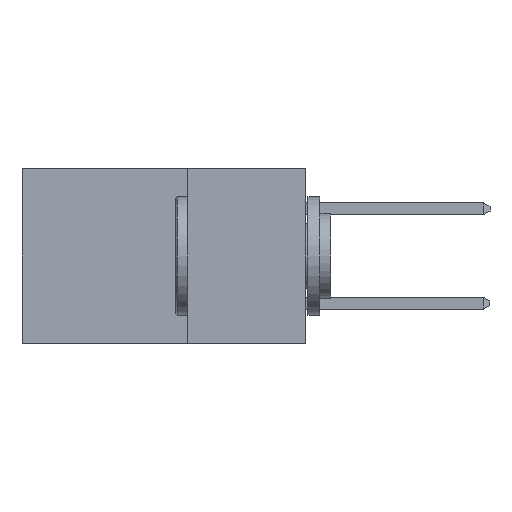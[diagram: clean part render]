
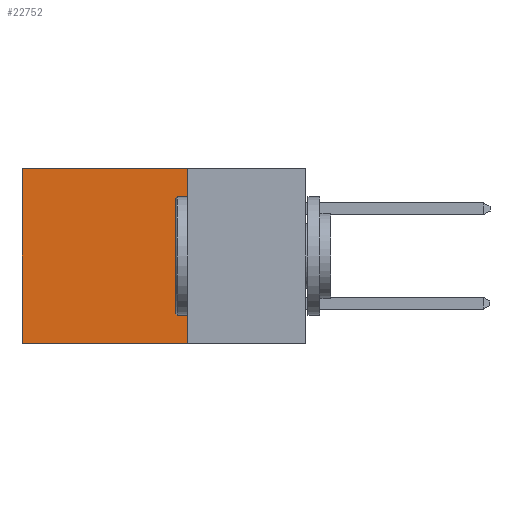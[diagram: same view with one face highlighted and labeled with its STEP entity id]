
A CAD part, left-side view. The second image highlights one B-rep face of the part: STEP entity #22752.
In plain terms, the highlighted planar face has unit normal (-1, 0, 0).
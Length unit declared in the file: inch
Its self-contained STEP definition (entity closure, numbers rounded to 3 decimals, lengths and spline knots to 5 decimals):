
#665 = LINE ( 'NONE', #20481, #9593 ) ;
#2445 = VERTEX_POINT ( 'NONE', #21911 ) ;
#3149 = LINE ( 'NONE', #11725, #16633 ) ;
#3581 = VERTEX_POINT ( 'NONE', #5821 ) ;
#3731 = EDGE_LOOP ( 'NONE', ( #21930, #4913, #4313, #12067 ) ) ;
#4313 = ORIENTED_EDGE ( 'NONE', *, *, #7236, .F. ) ;
#4332 = VERTEX_POINT ( 'NONE', #10172 ) ;
#4491 = DIRECTION ( 'NONE',  ( 1., 0., 0. ) ) ;
#4913 = ORIENTED_EDGE ( 'NONE', *, *, #10407, .F. ) ;
#5600 = EDGE_CURVE ( 'NONE', #4332, #2445, #18205, .T. ) ;
#5821 = CARTESIAN_POINT ( 'NONE',  ( 0.298, 0.25, -0.37 ) ) ;
#6002 = CARTESIAN_POINT ( 'NONE',  ( 0.298, 0.6, -0.37 ) ) ;
#6508 = VERTEX_POINT ( 'NONE', #6002 ) ;
#7236 = EDGE_CURVE ( 'NONE', #4332, #3581, #17273, .T. ) ;
#8006 = VECTOR ( 'NONE', #16005, 39.37008 ) ;
#8474 = EDGE_CURVE ( 'NONE', #2445, #6508, #665, .T. ) ;
#9593 = VECTOR ( 'NONE', #20512, 39.37008 ) ;
#9943 = AXIS2_PLACEMENT_3D ( 'NONE', #14978, #4491, #16739 ) ;
#10172 = CARTESIAN_POINT ( 'NONE',  ( 0.298, 0.25, 0. ) ) ;
#10407 = EDGE_CURVE ( 'NONE', #3581, #6508, #3149, .T. ) ;
#11006 = CARTESIAN_POINT ( 'NONE',  ( 0.298, 0.25, 0. ) ) ;
#11725 = CARTESIAN_POINT ( 'NONE',  ( 0.298, 0.25, -0.37 ) ) ;
#12067 = ORIENTED_EDGE ( 'NONE', *, *, #5600, .T. ) ;
#13514 = VECTOR ( 'NONE', #21735, 39.37008 ) ;
#13902 = FACE_OUTER_BOUND ( 'NONE', #3731, .T. ) ;
#14978 = CARTESIAN_POINT ( 'NONE',  ( 0.298, 0.25, 0. ) ) ;
#16005 = DIRECTION ( 'NONE',  ( 0., 0., -1. ) ) ;
#16633 = VECTOR ( 'NONE', #22367, 39.37008 ) ;
#16739 = DIRECTION ( 'NONE',  ( 0., 0., -1. ) ) ;
#17273 = LINE ( 'NONE', #17735, #8006 ) ;
#17735 = CARTESIAN_POINT ( 'NONE',  ( 0.298, 0.25, 0. ) ) ;
#18205 = LINE ( 'NONE', #11006, #13514 ) ;
#20481 = CARTESIAN_POINT ( 'NONE',  ( 0.298, 0.6, 0. ) ) ;
#20512 = DIRECTION ( 'NONE',  ( 0., 0., -1. ) ) ;
#21735 = DIRECTION ( 'NONE',  ( 0., 1., 0. ) ) ;
#21911 = CARTESIAN_POINT ( 'NONE',  ( 0.298, 0.6, 0. ) ) ;
#21930 = ORIENTED_EDGE ( 'NONE', *, *, #8474, .T. ) ;
#22015 = PLANE ( 'NONE',  #9943 ) ;
#22367 = DIRECTION ( 'NONE',  ( 0., 1., 0. ) ) ;
#22752 = ADVANCED_FACE ( 'NONE', ( #13902 ), #22015, .F. ) ;
